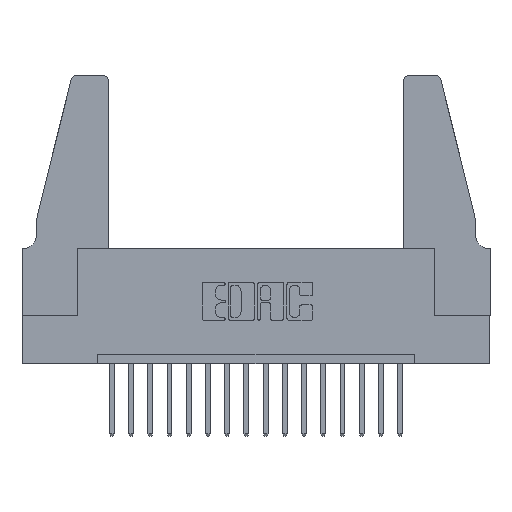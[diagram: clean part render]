
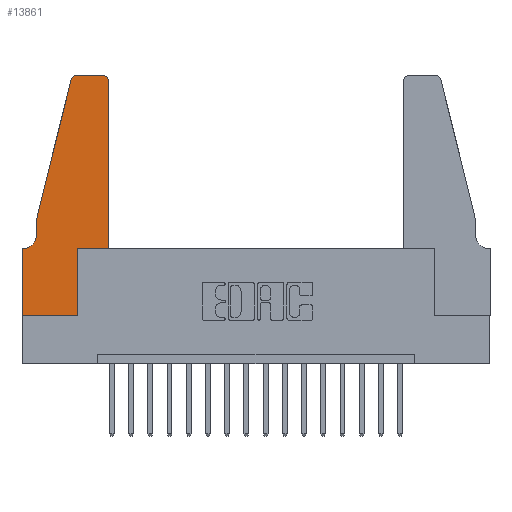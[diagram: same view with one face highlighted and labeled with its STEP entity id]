
A CAD part, top view. The second image highlights one B-rep face of the part: STEP entity #13861.
In plain terms, the highlighted planar face has unit normal (0, 0, 1).
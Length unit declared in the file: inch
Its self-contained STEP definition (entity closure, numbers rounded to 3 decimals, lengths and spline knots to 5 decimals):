
#333 = DIRECTION ( 'NONE',  ( -1., 0., 0. ) ) ;
#386 = DIRECTION ( 'NONE',  ( 0., 0., -1. ) ) ;
#404 = CARTESIAN_POINT ( 'NONE',  ( 0.0755, 0.5, 0.37 ) ) ;
#569 = ORIENTED_EDGE ( 'NONE', *, *, #7973, .T. ) ;
#812 = CARTESIAN_POINT ( 'NONE',  ( 0.0755, 0.5, 0.37 ) ) ;
#917 = DIRECTION ( 'NONE',  ( -1., 0., 0. ) ) ;
#1027 = DIRECTION ( 'NONE',  ( -0.239, -0.971, 0. ) ) ;
#1079 = DIRECTION ( 'NONE',  ( 1., 0., 0. ) ) ;
#1191 = CARTESIAN_POINT ( 'NONE',  ( 0.4505, 0.35, 0.37 ) ) ;
#1523 = CARTESIAN_POINT ( 'NONE',  ( 0.0755, 0.5, 0.37 ) ) ;
#1556 = VERTEX_POINT ( 'NONE', #9192 ) ;
#1732 = CARTESIAN_POINT ( 'NONE',  ( 0.4505, 1.22, 0.37 ) ) ;
#1734 = EDGE_LOOP ( 'NONE', ( #13009, #569, #13628, #2837, #5471, #17651, #12570, #13802, #8859, #2403, #2307, #15080 ) ) ;
#1793 = VERTEX_POINT ( 'NONE', #2959 ) ;
#2307 = ORIENTED_EDGE ( 'NONE', *, *, #6774, .T. ) ;
#2403 = ORIENTED_EDGE ( 'NONE', *, *, #4214, .T. ) ;
#2489 = LINE ( 'NONE', #1523, #16646 ) ;
#2837 = ORIENTED_EDGE ( 'NONE', *, *, #7558, .T. ) ;
#2959 = CARTESIAN_POINT ( 'NONE',  ( 0.284, 1.25, 0.37 ) ) ;
#3145 = LINE ( 'NONE', #13136, #7924 ) ;
#3178 = CARTESIAN_POINT ( 'NONE',  ( 0.4205, 1.25, 0.37 ) ) ;
#3348 = CIRCLE ( 'NONE', #11626, 0.03 ) ;
#3629 = DIRECTION ( 'NONE',  ( 1., 0., 0. ) ) ;
#3698 = VERTEX_POINT ( 'NONE', #4067 ) ;
#3801 = VECTOR ( 'NONE', #1027, 39.37008 ) ;
#3861 = VERTEX_POINT ( 'NONE', #1732 ) ;
#3889 = PLANE ( 'NONE',  #11708 ) ;
#4010 = DIRECTION ( 'NONE',  ( 1., 0., 0. ) ) ;
#4067 = CARTESIAN_POINT ( 'NONE',  ( 0., 0., 0.37 ) ) ;
#4214 = EDGE_CURVE ( 'NONE', #12150, #1556, #3145, .T. ) ;
#4615 = VERTEX_POINT ( 'NONE', #3178 ) ;
#4942 = VECTOR ( 'NONE', #17713, 39.37008 ) ;
#5039 = CARTESIAN_POINT ( 'NONE',  ( 0.0755, 0.35, 0.37 ) ) ;
#5094 = DIRECTION ( 'NONE',  ( 0., 0., 1. ) ) ;
#5306 = AXIS2_PLACEMENT_3D ( 'NONE', #6254, #7649, #9021 ) ;
#5332 = DIRECTION ( 'NONE',  ( 0., 1., 0. ) ) ;
#5471 = ORIENTED_EDGE ( 'NONE', *, *, #10825, .T. ) ;
#5725 = VERTEX_POINT ( 'NONE', #404 ) ;
#5947 = VECTOR ( 'NONE', #917, 39.37008 ) ;
#6187 = LINE ( 'NONE', #8189, #14068 ) ;
#6212 = CARTESIAN_POINT ( 'NONE',  ( 0.0755, 0.42, 0.37 ) ) ;
#6254 = CARTESIAN_POINT ( 'NONE',  ( 0.4205, 1.22, 0.37 ) ) ;
#6558 = DIRECTION ( 'NONE',  ( 0., 0., 1. ) ) ;
#6710 = CARTESIAN_POINT ( 'NONE',  ( 0.2865, 0.35, 0.37 ) ) ;
#6774 = EDGE_CURVE ( 'NONE', #1556, #3861, #15192, .T. ) ;
#6884 = VERTEX_POINT ( 'NONE', #12353 ) ;
#6926 = DIRECTION ( 'NONE',  ( 0., -1., 0. ) ) ;
#7267 = VECTOR ( 'NONE', #4010, 39.37008 ) ;
#7558 = EDGE_CURVE ( 'NONE', #5725, #13643, #2489, .T. ) ;
#7564 = EDGE_CURVE ( 'NONE', #14154, #3698, #6187, .T. ) ;
#7649 = DIRECTION ( 'NONE',  ( 0., 0., 1. ) ) ;
#7918 = LINE ( 'NONE', #9358, #7267 ) ;
#7924 = VECTOR ( 'NONE', #3629, 39.37008 ) ;
#7945 = EDGE_CURVE ( 'NONE', #10174, #5725, #9823, .T. ) ;
#7973 = EDGE_CURVE ( 'NONE', #1793, #10174, #3348, .T. ) ;
#8189 = CARTESIAN_POINT ( 'NONE',  ( 0., 0., 0.37 ) ) ;
#8585 = VECTOR ( 'NONE', #10621, 39.37008 ) ;
#8859 = ORIENTED_EDGE ( 'NONE', *, *, #17008, .T. ) ;
#9021 = DIRECTION ( 'NONE',  ( 1., 0., 0. ) ) ;
#9192 = CARTESIAN_POINT ( 'NONE',  ( 0.4505, 0.35, 0.37 ) ) ;
#9358 = CARTESIAN_POINT ( 'NONE',  ( 0., 0., 0.37 ) ) ;
#9616 = DIRECTION ( 'NONE',  ( 0., -1., 0. ) ) ;
#9823 = LINE ( 'NONE', #812, #3801 ) ;
#10174 = VERTEX_POINT ( 'NONE', #15679 ) ;
#10258 = CARTESIAN_POINT ( 'NONE',  ( 0.0055, 0.35, 0.37 ) ) ;
#10492 = CARTESIAN_POINT ( 'NONE',  ( 0.284, 1.22, 0.37 ) ) ;
#10621 = DIRECTION ( 'NONE',  ( -1., 0., 0. ) ) ;
#10735 = CARTESIAN_POINT ( 'NONE',  ( 0.2605, 1.25, 0.37 ) ) ;
#10825 = EDGE_CURVE ( 'NONE', #13643, #14859, #17156, .T. ) ;
#11162 = LINE ( 'NONE', #6710, #4942 ) ;
#11626 = AXIS2_PLACEMENT_3D ( 'NONE', #10492, #6558, #16085 ) ;
#11708 = AXIS2_PLACEMENT_3D ( 'NONE', #14717, #5094, #1079 ) ;
#12150 = VERTEX_POINT ( 'NONE', #15117 ) ;
#12313 = CIRCLE ( 'NONE', #5306, 0.03 ) ;
#12353 = CARTESIAN_POINT ( 'NONE',  ( 0.2865, 0., 0.37 ) ) ;
#12556 = LINE ( 'NONE', #5039, #5947 ) ;
#12570 = ORIENTED_EDGE ( 'NONE', *, *, #7564, .T. ) ;
#13009 = ORIENTED_EDGE ( 'NONE', *, *, #17486, .T. ) ;
#13041 = LINE ( 'NONE', #10735, #8585 ) ;
#13134 = EDGE_CURVE ( 'NONE', #3698, #6884, #7918, .T. ) ;
#13136 = CARTESIAN_POINT ( 'NONE',  ( 0.4505, 0.35, 0.37 ) ) ;
#13495 = EDGE_CURVE ( 'NONE', #14859, #14154, #12556, .T. ) ;
#13628 = ORIENTED_EDGE ( 'NONE', *, *, #7945, .T. ) ;
#13643 = VERTEX_POINT ( 'NONE', #6212 ) ;
#13802 = ORIENTED_EDGE ( 'NONE', *, *, #13134, .T. ) ;
#13861 = ADVANCED_FACE ( 'NONE', ( #17674 ), #3889, .T. ) ;
#13968 = EDGE_CURVE ( 'NONE', #3861, #4615, #12313, .T. ) ;
#14068 = VECTOR ( 'NONE', #6926, 39.37008 ) ;
#14154 = VERTEX_POINT ( 'NONE', #15743 ) ;
#14326 = VECTOR ( 'NONE', #5332, 39.37008 ) ;
#14717 = CARTESIAN_POINT ( 'NONE',  ( 0., 0.35, 0.37 ) ) ;
#14859 = VERTEX_POINT ( 'NONE', #10258 ) ;
#15080 = ORIENTED_EDGE ( 'NONE', *, *, #13968, .T. ) ;
#15117 = CARTESIAN_POINT ( 'NONE',  ( 0.2865, 0.35, 0.37 ) ) ;
#15192 = LINE ( 'NONE', #1191, #14326 ) ;
#15322 = CARTESIAN_POINT ( 'NONE',  ( 0.0055, 0.42, 0.37 ) ) ;
#15679 = CARTESIAN_POINT ( 'NONE',  ( 0.25487, 1.22718, 0.37 ) ) ;
#15743 = CARTESIAN_POINT ( 'NONE',  ( 0., 0.35, 0.37 ) ) ;
#16085 = DIRECTION ( 'NONE',  ( 1., 0., 0. ) ) ;
#16646 = VECTOR ( 'NONE', #9616, 39.37008 ) ;
#17003 = AXIS2_PLACEMENT_3D ( 'NONE', #15322, #386, #333 ) ;
#17008 = EDGE_CURVE ( 'NONE', #6884, #12150, #11162, .T. ) ;
#17156 = CIRCLE ( 'NONE', #17003, 0.07 ) ;
#17486 = EDGE_CURVE ( 'NONE', #4615, #1793, #13041, .T. ) ;
#17651 = ORIENTED_EDGE ( 'NONE', *, *, #13495, .T. ) ;
#17674 = FACE_OUTER_BOUND ( 'NONE', #1734, .T. ) ;
#17713 = DIRECTION ( 'NONE',  ( 0., 1., 0. ) ) ;
